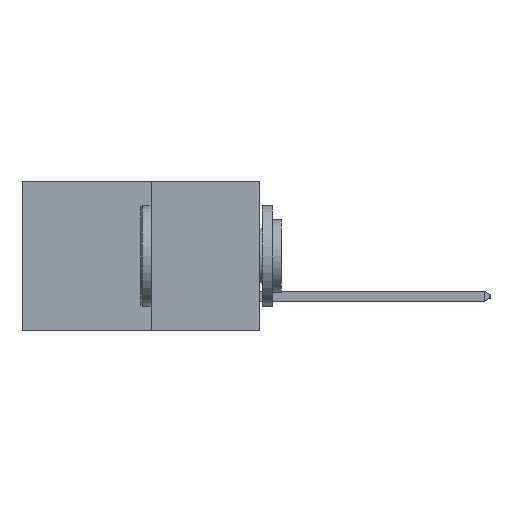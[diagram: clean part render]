
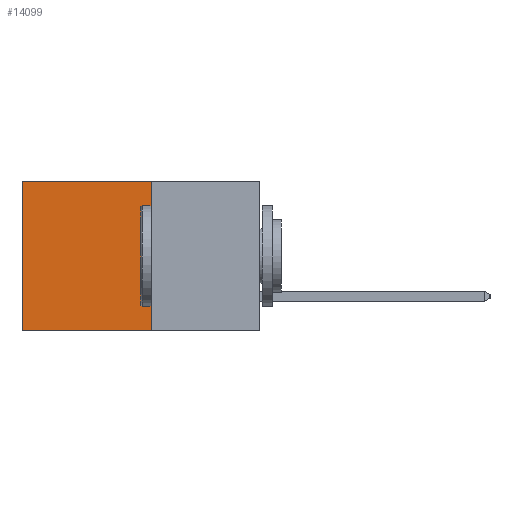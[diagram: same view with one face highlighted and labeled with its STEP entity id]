
A CAD part, left-side view. The second image highlights one B-rep face of the part: STEP entity #14099.
In plain terms, the highlighted planar face has unit normal (-1, 0, 0).
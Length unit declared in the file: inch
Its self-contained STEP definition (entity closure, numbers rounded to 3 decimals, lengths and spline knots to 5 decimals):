
#322 = DIRECTION ( 'NONE',  ( 0., 0., -1. ) ) ;
#722 = VERTEX_POINT ( 'NONE', #13660 ) ;
#775 = EDGE_LOOP ( 'NONE', ( #8826, #1275, #14656, #2033 ) ) ;
#1275 = ORIENTED_EDGE ( 'NONE', *, *, #2302, .F. ) ;
#1951 = VECTOR ( 'NONE', #13070, 39.37008 ) ;
#2018 = LINE ( 'NONE', #5056, #8141 ) ;
#2033 = ORIENTED_EDGE ( 'NONE', *, *, #6409, .T. ) ;
#2302 = EDGE_CURVE ( 'NONE', #7706, #722, #8078, .T. ) ;
#3095 = AXIS2_PLACEMENT_3D ( 'NONE', #13910, #7258, #322 ) ;
#4920 = CARTESIAN_POINT ( 'NONE',  ( 0.277, 0.27, -0.37 ) ) ;
#5056 = CARTESIAN_POINT ( 'NONE',  ( 0.277, 0.59, -0.37 ) ) ;
#5118 = VECTOR ( 'NONE', #7561, 39.37008 ) ;
#5181 = CARTESIAN_POINT ( 'NONE',  ( 0.277, 0.59, 0. ) ) ;
#6409 = EDGE_CURVE ( 'NONE', #12721, #12301, #11177, .T. ) ;
#7258 = DIRECTION ( 'NONE',  ( 1., 0., 0. ) ) ;
#7561 = DIRECTION ( 'NONE',  ( 0., 1., 0. ) ) ;
#7609 = CARTESIAN_POINT ( 'NONE',  ( 0.277, 0.27, 0. ) ) ;
#7706 = VERTEX_POINT ( 'NONE', #12625 ) ;
#7761 = VECTOR ( 'NONE', #11707, 39.37008 ) ;
#8078 = LINE ( 'NONE', #12869, #1951 ) ;
#8141 = VECTOR ( 'NONE', #8545, 39.37008 ) ;
#8271 = CARTESIAN_POINT ( 'NONE',  ( 0.277, 0.27, 0. ) ) ;
#8545 = DIRECTION ( 'NONE',  ( 0., 0., -1. ) ) ;
#8826 = ORIENTED_EDGE ( 'NONE', *, *, #9378, .T. ) ;
#8859 = FACE_OUTER_BOUND ( 'NONE', #775, .T. ) ;
#9378 = EDGE_CURVE ( 'NONE', #12301, #722, #2018, .T. ) ;
#11177 = LINE ( 'NONE', #7609, #5118 ) ;
#11707 = DIRECTION ( 'NONE',  ( 0., 0., -1. ) ) ;
#11719 = PLANE ( 'NONE',  #3095 ) ;
#12301 = VERTEX_POINT ( 'NONE', #5181 ) ;
#12625 = CARTESIAN_POINT ( 'NONE',  ( 0.277, 0.27, -0.37 ) ) ;
#12721 = VERTEX_POINT ( 'NONE', #8271 ) ;
#12869 = CARTESIAN_POINT ( 'NONE',  ( 0.277, 0.27, -0.37 ) ) ;
#13070 = DIRECTION ( 'NONE',  ( 0., 1., 0. ) ) ;
#13645 = LINE ( 'NONE', #4920, #7761 ) ;
#13660 = CARTESIAN_POINT ( 'NONE',  ( 0.277, 0.59, -0.37 ) ) ;
#13910 = CARTESIAN_POINT ( 'NONE',  ( 0.277, 0.27, -0.37 ) ) ;
#14099 = ADVANCED_FACE ( 'NONE', ( #8859 ), #11719, .F. ) ;
#14608 = EDGE_CURVE ( 'NONE', #12721, #7706, #13645, .T. ) ;
#14656 = ORIENTED_EDGE ( 'NONE', *, *, #14608, .F. ) ;
